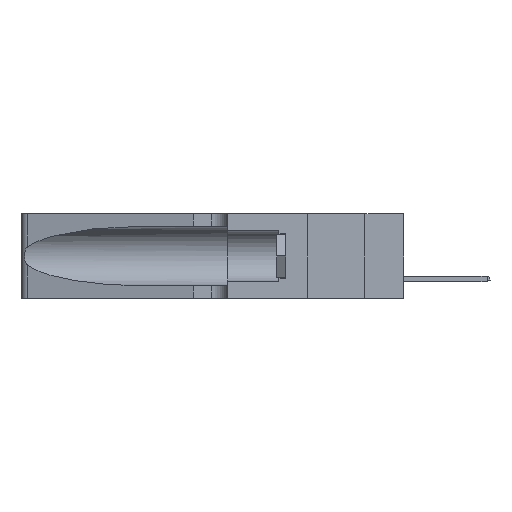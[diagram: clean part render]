
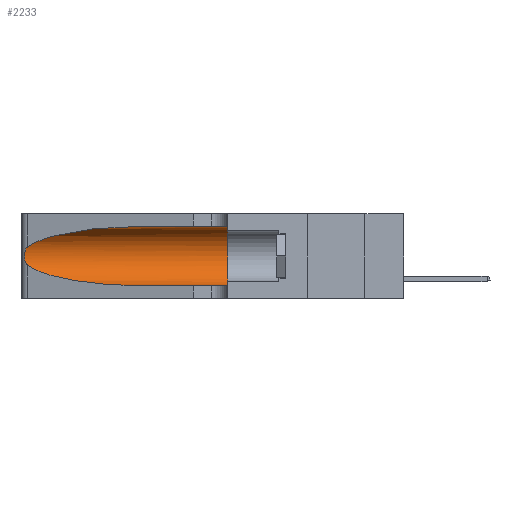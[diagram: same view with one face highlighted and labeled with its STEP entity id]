
A CAD part, left-side view. The second image highlights one B-rep face of the part: STEP entity #2233.
In plain terms, the highlighted cylindrical face has radius 3.308 mm (diameter 6.617 mm), a partial arc.
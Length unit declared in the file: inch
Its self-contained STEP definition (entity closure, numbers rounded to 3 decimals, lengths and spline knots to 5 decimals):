
#596 = CARTESIAN_POINT ( 'NONE',  ( 0.25854, 1.2359, 0.20912 ) ) ;
#864 = DIRECTION ( 'NONE',  ( 0., 1., 0. ) ) ;
#1250 = VERTEX_POINT ( 'NONE', #8579 ) ;
#1291 = CARTESIAN_POINT ( 'NONE',  ( 0.1305, 1.61858, 0.05475 ) ) ;
#2233 = ADVANCED_FACE ( 'NONE', ( #16482 ), #15992, .F. ) ;
#2324 = VERTEX_POINT ( 'NONE', #21067 ) ;
#3021 = CARTESIAN_POINT ( 'NONE',  ( 0.25555, 1.22994, 0.2215 ) ) ;
#3254 = CARTESIAN_POINT ( 'NONE',  ( 0.25639, 1.23184, 0.21858 ) ) ;
#3499 = CARTESIAN_POINT ( 'NONE',  ( 0.26075, 1.23896, 0.19203 ) ) ;
#3652 = CARTESIAN_POINT ( 'NONE',  ( 0.25487, 1.22718, 0.22369 ) ) ;
#6369 = CARTESIAN_POINT ( 'NONE',  ( 0.25555, 1.22993, 0.14849 ) ) ;
#6634 = EDGE_CURVE ( 'NONE', #23148, #1250, #20077, .T. ) ;
#7100 = AXIS2_PLACEMENT_3D ( 'NONE', #20834, #11912, #15271 ) ;
#7227 = CARTESIAN_POINT ( 'NONE',  ( 0.25487, 1.22718, 0.14631 ) ) ;
#8038 = VERTEX_POINT ( 'NONE', #19975 ) ;
#8396 = VECTOR ( 'NONE', #10174, 39.37008 ) ;
#8579 = CARTESIAN_POINT ( 'NONE',  ( 0.1305, 0.35, 0.05475 ) ) ;
#9023 = EDGE_CURVE ( 'NONE', #2324, #16487, #16661, .T. ) ;
#9253 = CARTESIAN_POINT ( 'NONE',  ( 0.25639, 1.23186, 0.15144 ) ) ;
#9525 = ORIENTED_EDGE ( 'NONE', *, *, #9023, .T. ) ;
#9933 = CARTESIAN_POINT ( 'NONE',  ( 0.1305, 1.61858, 0.31525 ) ) ;
#10133 = EDGE_CURVE ( 'NONE', #8038, #33382, #20063, .T. ) ;
#10174 = DIRECTION ( 'NONE',  ( 0., -1., 0. ) ) ;
#10237 = CARTESIAN_POINT ( 'NONE',  ( 0.2373, 1.15595, 0.08982 ) ) ;
#10533 = CARTESIAN_POINT ( 'NONE',  ( 0.1305, 0.72297, 0.31525 ) ) ;
#11912 = DIRECTION ( 'NONE',  ( 0., -1., 0. ) ) ;
#12650 = CARTESIAN_POINT ( 'NONE',  ( 0.25789, 1.23486, 0.15765 ) ) ;
#13341 = ORIENTED_EDGE ( 'NONE', *, *, #35727, .T. ) ;
#13743 = DIRECTION ( 'NONE',  ( 0., 0., 1. ) ) ;
#15271 = DIRECTION ( 'NONE',  ( 0., 0., -1. ) ) ;
#15322 = ORIENTED_EDGE ( 'NONE', *, *, #21632, .T. ) ;
#15418 = CARTESIAN_POINT ( 'NONE',  ( 0.25856, 1.23593, 0.16098 ) ) ;
#15606 = CARTESIAN_POINT ( 'NONE',  ( 0.1305, 0.35, 0.31525 ) ) ;
#15960 = ORIENTED_EDGE ( 'NONE', *, *, #6634, .F. ) ;
#15992 = CYLINDRICAL_SURFACE ( 'NONE', #7100, 0.13025 ) ;
#16482 = FACE_OUTER_BOUND ( 'NONE', #31543, .T. ) ;
#16487 = VERTEX_POINT ( 'NONE', #3652 ) ;
#16644 = CARTESIAN_POINT ( 'NONE',  ( 0.1305, 0.72297, 0.05475 ) ) ;
#16661 =( BOUNDED_CURVE ( )  B_SPLINE_CURVE ( 3, ( #10533, #25817, #26084, #28923 ),
 .UNSPECIFIED., .F., .F. ) 
 B_SPLINE_CURVE_WITH_KNOTS ( ( 4, 4 ),
 ( 1.5708, 2.84003 ),
 .UNSPECIFIED. ) 
 CURVE ( )  GEOMETRIC_REPRESENTATION_ITEM ( )  RATIONAL_B_SPLINE_CURVE ( ( 1., 0.87, 0.87, 1. ) ) 
 REPRESENTATION_ITEM ( '' )  );
#17964 = CARTESIAN_POINT ( 'NONE',  ( 0.25487, 1.22718, 0.22369 ) ) ;
#18436 = CARTESIAN_POINT ( 'NONE',  ( 0.26017, 1.23833, 0.17102 ) ) ;
#18822 = CARTESIAN_POINT ( 'NONE',  ( 0.1305, 0.35, 0.185 ) ) ;
#19537 = B_SPLINE_CURVE_WITH_KNOTS ( 'NONE', 3,
 ( #17964, #3021, #3254, #30637, #596, #24360, #3499, #36527, #18436, #15418, #12650, #9253, #6369, #21578 ),
 .UNSPECIFIED., .F., .F.,
 ( 4, 2, 2, 2, 2, 2, 4 ),
 ( 0., 0.00027, 0.00053, 0.00107, 0.0016, 0.00187, 0.00214 ),
 .UNSPECIFIED. ) ;
#19975 = CARTESIAN_POINT ( 'NONE',  ( 0.25487, 1.22718, 0.14631 ) ) ;
#20063 =( BOUNDED_CURVE ( )  B_SPLINE_CURVE ( 3, ( #7227, #10237, #30886, #16644 ),
 .UNSPECIFIED., .F., .T. ) 
 B_SPLINE_CURVE_WITH_KNOTS ( ( 4, 4 ),
 ( 3.44316, 4.71239 ),
 .UNSPECIFIED. ) 
 CURVE ( )  GEOMETRIC_REPRESENTATION_ITEM ( )  RATIONAL_B_SPLINE_CURVE ( ( 1., 0.87, 0.87, 1. ) ) 
 REPRESENTATION_ITEM ( '' )  );
#20077 = CIRCLE ( 'NONE', #31059, 0.13025 ) ;
#20834 = CARTESIAN_POINT ( 'NONE',  ( 0.1305, 1.61858, 0.185 ) ) ;
#21067 = CARTESIAN_POINT ( 'NONE',  ( 0.1305, 0.72297, 0.31525 ) ) ;
#21578 = CARTESIAN_POINT ( 'NONE',  ( 0.25487, 1.22718, 0.14631 ) ) ;
#21632 = EDGE_CURVE ( 'NONE', #33382, #1250, #33214, .T. ) ;
#22014 = DIRECTION ( 'NONE',  ( 0., -1., 0. ) ) ;
#22800 = ORIENTED_EDGE ( 'NONE', *, *, #28343, .F. ) ;
#23148 = VERTEX_POINT ( 'NONE', #15606 ) ;
#23260 = ORIENTED_EDGE ( 'NONE', *, *, #10133, .T. ) ;
#24360 = CARTESIAN_POINT ( 'NONE',  ( 0.26018, 1.23835, 0.19895 ) ) ;
#24551 = VECTOR ( 'NONE', #22014, 39.37008 ) ;
#25817 = CARTESIAN_POINT ( 'NONE',  ( 0.18966, 0.96281, 0.31525 ) ) ;
#26084 = CARTESIAN_POINT ( 'NONE',  ( 0.2373, 1.15595, 0.28018 ) ) ;
#28343 = EDGE_CURVE ( 'NONE', #2324, #23148, #31622, .T. ) ;
#28923 = CARTESIAN_POINT ( 'NONE',  ( 0.25487, 1.22718, 0.22369 ) ) ;
#30637 = CARTESIAN_POINT ( 'NONE',  ( 0.25787, 1.23484, 0.2124 ) ) ;
#30886 = CARTESIAN_POINT ( 'NONE',  ( 0.18966, 0.96281, 0.05475 ) ) ;
#31059 = AXIS2_PLACEMENT_3D ( 'NONE', #18822, #864, #13743 ) ;
#31543 = EDGE_LOOP ( 'NONE', ( #9525, #13341, #23260, #15322, #15960, #22800 ) ) ;
#31622 = LINE ( 'NONE', #9933, #24551 ) ;
#33214 = LINE ( 'NONE', #1291, #8396 ) ;
#33382 = VERTEX_POINT ( 'NONE', #34630 ) ;
#34630 = CARTESIAN_POINT ( 'NONE',  ( 0.1305, 0.72297, 0.05475 ) ) ;
#35727 = EDGE_CURVE ( 'NONE', #16487, #8038, #19537, .T. ) ;
#36527 = CARTESIAN_POINT ( 'NONE',  ( 0.26075, 1.23896, 0.178 ) ) ;
